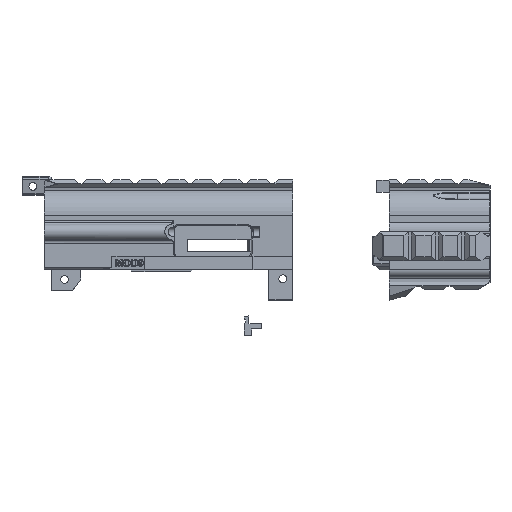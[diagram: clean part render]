
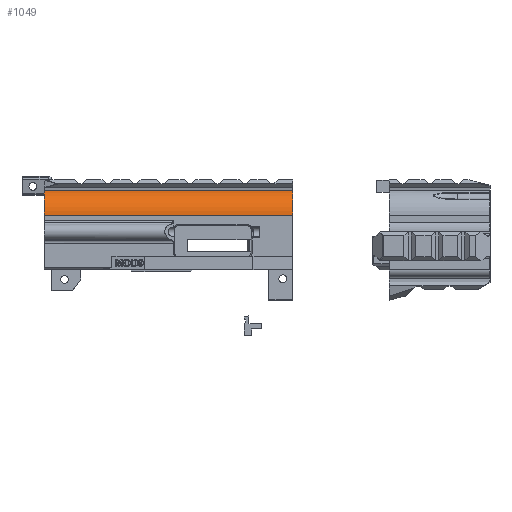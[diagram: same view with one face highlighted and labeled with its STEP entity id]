
A CAD part, top view. The second image highlights one B-rep face of the part: STEP entity #1049.
In plain terms, the highlighted cylindrical face has radius 20.1 mm (diameter 40.2 mm), a partial arc.
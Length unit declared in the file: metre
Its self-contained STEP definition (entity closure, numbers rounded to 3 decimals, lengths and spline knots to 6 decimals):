
#1049=ADVANCED_FACE('3023:8280',(#3210),#3211,.T.);
#3210=FACE_OUTER_BOUND('',#7004,.T.);
#3211=CYLINDRICAL_SURFACE('',#7005,0.0201);
#7004=EDGE_LOOP('',(#15985,#15986,#15987,#15988));
#7005=AXIS2_PLACEMENT_3D('',#15989,#15990,#15991);
#15985=ORIENTED_EDGE('',*,*,#21380,.T.);
#15986=ORIENTED_EDGE('',*,*,#21168,.T.);
#15987=ORIENTED_EDGE('',*,*,#21379,.F.);
#15988=ORIENTED_EDGE('',*,*,#21303,.T.);
#15989=CARTESIAN_POINT('',(-0.020072,0.047361,0.001));
#15990=DIRECTION('',(1.0,0.,0.));
#15991=DIRECTION('',(0.,0.,-1.0));
#21168=EDGE_CURVE('3023:10914',#26256,#26254,#26257,.T.);
#21303=EDGE_CURVE('3023:11319',#26481,#26479,#26482,.T.);
#21379=EDGE_CURVE('3023:11547',#26481,#26254,#26595,.T.);
#21380=EDGE_CURVE('3023:11550',#26479,#26256,#26596,.T.);
#26254=VERTEX_POINT('',#36162);
#26256=VERTEX_POINT('',#36165);
#26257=CIRCLE('',#36166,0.0201);
#26479=VERTEX_POINT('',#36502);
#26481=VERTEX_POINT('',#36505);
#26482=CIRCLE('',#36506,0.0201);
#26595=LINE('',#36688,#36689);
#26596=LINE('',#36690,#36691);
#36162=CARTESIAN_POINT('',(-0.178704,0.047361,0.0211));
#36165=CARTESIAN_POINT('',(-0.178704,0.065991,0.008545));
#36166=AXIS2_PLACEMENT_3D('',#43047,#43048,#43049);
#36502=CARTESIAN_POINT('',(0.011678,0.065991,0.008545));
#36505=CARTESIAN_POINT('',(0.011678,0.047361,0.0211));
#36506=AXIS2_PLACEMENT_3D('',#43229,#43230,#43231);
#36688=CARTESIAN_POINT('',(-0.020072,0.047361,0.0211));
#36689=VECTOR('',#43319,0.190382);
#36690=CARTESIAN_POINT('',(-0.020072,0.065991,0.008545));
#36691=VECTOR('',#43320,0.190382);
#43047=CARTESIAN_POINT('',(-0.178704,0.047361,0.001));
#43048=DIRECTION('',(1.0,0.,0.));
#43049=DIRECTION('',(0.,0.,-1.0));
#43229=CARTESIAN_POINT('',(0.011678,0.047361,0.001));
#43230=DIRECTION('',(-1.0,0.,0.));
#43231=DIRECTION('',(0.,0.,-1.0));
#43319=DIRECTION('',(-1.0,0.0,0.));
#43320=DIRECTION('',(-1.0,0.0,0.));
